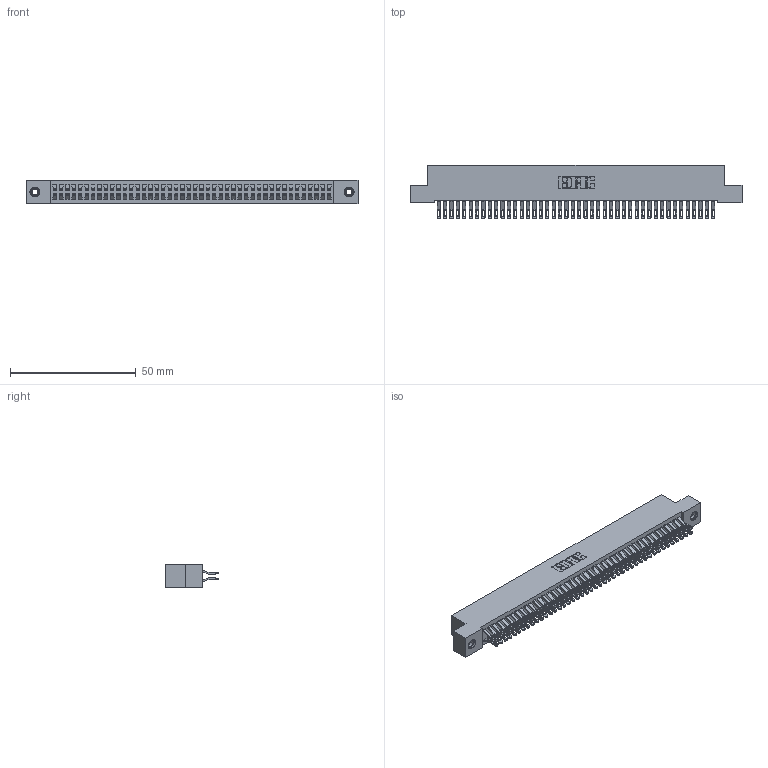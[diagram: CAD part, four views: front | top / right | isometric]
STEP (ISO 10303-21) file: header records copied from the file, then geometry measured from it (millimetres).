
FILE_DESCRIPTION (( 'STEP AP203' ), '1' );
FILE_NAME ('392-088-555-208.STEP', '2018-08-18T06:24:30', ( '' ), ( '' ), 'SwSTEP 2.0', 'SolidWorks 2016', '' );
FILE_SCHEMA (( 'CONFIG_CONTROL_DESIGN' ));
Length unit declared in the file: inch
Products named in the file (4): 342 Part_TI; 345-292-001_555 Tail; 345-250-001_345-250-003-102; 392-088-555-208
Assembly tree (91 placements, depth 2):
  392-088-555-208
    342 Part_TI
    345-292-001_555 Tail  x88
    345-250-001_345-250-003-102  x2
Bounding box: 132.08 x 21.47 x 9.4 mm (x, y, z)
Volume: 12115.7 mm3; surface area: 20632.3 mm2
Topology: 91 solids, 91 shells, 5274 faces, 16539 edges, 11018 vertices
Faces by surface type: plane 3090, cylinder 2168, cone 12, torus 4
Entity records: 29428 total; most frequent: CARTESIAN_POINT 4891, ORIENTED_EDGE 4790, DIRECTION 4177, EDGE_CURVE 2395, LINE 2227, VECTOR 2227, VERTEX_POINT 1592, AXIS2_PLACEMENT_3D 975
